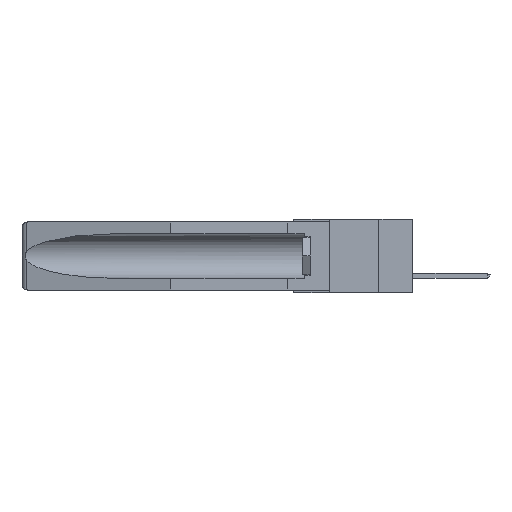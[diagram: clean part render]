
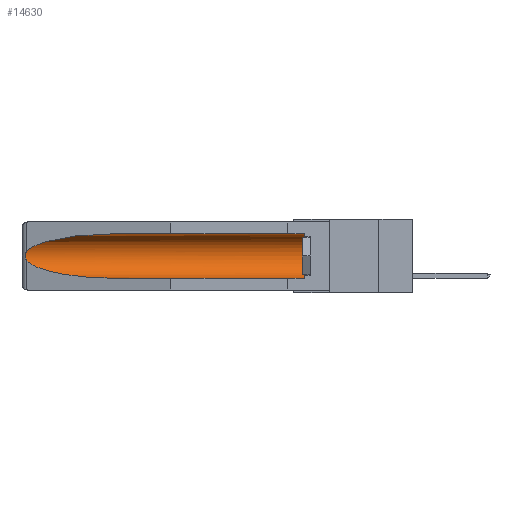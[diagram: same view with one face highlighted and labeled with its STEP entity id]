
A CAD part, left-side view. The second image highlights one B-rep face of the part: STEP entity #14630.
In plain terms, the highlighted cylindrical face has radius 2.857 mm (diameter 5.715 mm), a partial arc.
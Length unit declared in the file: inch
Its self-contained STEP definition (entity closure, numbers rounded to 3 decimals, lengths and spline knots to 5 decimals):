
#13 = CARTESIAN_POINT ( 'NONE',  ( 0.26537, 1.52718, -0.19328 ) ) ;
#518 = DIRECTION ( 'NONE',  ( 0., 0., 1. ) ) ;
#822 = CARTESIAN_POINT ( 'NONE',  ( 0.155, -0.30754, -0.1715 ) ) ;
#1220 = VECTOR ( 'NONE', #3973, 39.37008 ) ;
#1256 = CARTESIAN_POINT ( 'NONE',  ( 0.26537, 1.52718, -0.14972 ) ) ;
#1940 = ORIENTED_EDGE ( 'NONE', *, *, #6004, .T. ) ;
#2351 = ORIENTED_EDGE ( 'NONE', *, *, #6727, .T. ) ;
#2873 = CARTESIAN_POINT ( 'NONE',  ( 0.155, 1.07973, -0.059 ) ) ;
#3004 = CARTESIAN_POINT ( 'NONE',  ( 0.2675, 1.53308, -0.16763 ) ) ;
#3488 = CIRCLE ( 'NONE', #17014, 0.1125 ) ;
#3973 = DIRECTION ( 'NONE',  ( 0., 1., 0. ) ) ;
#4448 = VERTEX_POINT ( 'NONE', #9307 ) ;
#4563 = CARTESIAN_POINT ( 'NONE',  ( 0.26597, 1.52961, -0.15275 ) ) ;
#4626 = CARTESIAN_POINT ( 'NONE',  ( 0.2673, 1.53269, -0.17917 ) ) ;
#4885 = FACE_OUTER_BOUND ( 'NONE', #11073, .T. ) ;
#5135 = LINE ( 'NONE', #11339, #1220 ) ;
#5980 = CARTESIAN_POINT ( 'NONE',  ( 0.26537, 1.52718, -0.19328 ) ) ;
#6004 = EDGE_CURVE ( 'NONE', #4448, #8619, #3488, .T. ) ;
#6390 = CARTESIAN_POINT ( 'NONE',  ( 0.155, 1.07973, -0.284 ) ) ;
#6418 = ORIENTED_EDGE ( 'NONE', *, *, #13402, .T. ) ;
#6426 = CARTESIAN_POINT ( 'NONE',  ( 0.155, 1.07973, -0.284 ) ) ;
#6449 = CARTESIAN_POINT ( 'NONE',  ( 0.21114, 1.30732, -0.284 ) ) ;
#6727 = EDGE_CURVE ( 'NONE', #12605, #17943, #7594, .T. ) ;
#7241 = VERTEX_POINT ( 'NONE', #6426 ) ;
#7555 = CARTESIAN_POINT ( 'NONE',  ( 0.26597, 1.5296, -0.19026 ) ) ;
#7594 = B_SPLINE_CURVE_WITH_KNOTS ( 'NONE', 3,
 ( #7618, #4563, #14870, #11844, #3004, #16428, #4626, #16356, #7555, #5980 ),
 .UNSPECIFIED., .F., .F.,
 ( 4, 2, 2, 2, 4 ),
 ( 0., 0.00029, 0.00058, 0.00087, 0.00117 ),
 .UNSPECIFIED. ) ;
#7618 = CARTESIAN_POINT ( 'NONE',  ( 0.26537, 1.52718, -0.14972 ) ) ;
#8001 = VECTOR ( 'NONE', #18044, 39.37008 ) ;
#8006 = CARTESIAN_POINT ( 'NONE',  ( 0.26537, 1.52718, -0.19328 ) ) ;
#8587 = VERTEX_POINT ( 'NONE', #12379 ) ;
#8619 = VERTEX_POINT ( 'NONE', #9876 ) ;
#8806 = CARTESIAN_POINT ( 'NONE',  ( 0.26537, 1.52718, -0.14972 ) ) ;
#8815 = CYLINDRICAL_SURFACE ( 'NONE', #12055, 0.1125 ) ;
#9232 = CARTESIAN_POINT ( 'NONE',  ( 0.155, 0.126, -0.1715 ) ) ;
#9307 = CARTESIAN_POINT ( 'NONE',  ( 0.155, 0.126, -0.284 ) ) ;
#9475 = EDGE_CURVE ( 'NONE', #4448, #7241, #15582, .T. ) ;
#9541 = EDGE_CURVE ( 'NONE', #17943, #7241, #14062, .T. ) ;
#9876 = CARTESIAN_POINT ( 'NONE',  ( 0.155, 0.126, -0.059 ) ) ;
#10821 = DIRECTION ( 'NONE',  ( 0., -1., 0. ) ) ;
#11073 = EDGE_LOOP ( 'NONE', ( #6418, #2351, #15085, #17212, #1940, #13129 ) ) ;
#11310 = DIRECTION ( 'NONE',  ( 0., 0., 1. ) ) ;
#11339 = CARTESIAN_POINT ( 'NONE',  ( 0.155, -0.30754, -0.059 ) ) ;
#11844 = CARTESIAN_POINT ( 'NONE',  ( 0.2673, 1.5327, -0.16383 ) ) ;
#12055 = AXIS2_PLACEMENT_3D ( 'NONE', #822, #17046, #11310 ) ;
#12379 = CARTESIAN_POINT ( 'NONE',  ( 0.155, 1.07973, -0.059 ) ) ;
#12605 = VERTEX_POINT ( 'NONE', #1256 ) ;
#13129 = ORIENTED_EDGE ( 'NONE', *, *, #14238, .T. ) ;
#13402 = EDGE_CURVE ( 'NONE', #8587, #12605, #16166, .T. ) ;
#14062 =( BOUNDED_CURVE ( )  B_SPLINE_CURVE ( 3, ( #8006, #15325, #6449, #6390 ),
 .UNSPECIFIED., .F., .F. ) 
 B_SPLINE_CURVE_WITH_KNOTS ( ( 4, 4 ),
 ( 0.1948, 1.5708 ),
 .UNSPECIFIED. ) 
 CURVE ( )  GEOMETRIC_REPRESENTATION_ITEM ( )  RATIONAL_B_SPLINE_CURVE ( ( 1., 0.848, 0.848, 1. ) ) 
 REPRESENTATION_ITEM ( '' )  );
#14238 = EDGE_CURVE ( 'NONE', #8619, #8587, #5135, .T. ) ;
#14525 = CARTESIAN_POINT ( 'NONE',  ( 0.21114, 1.30732, -0.059 ) ) ;
#14630 = ADVANCED_FACE ( 'NONE', ( #4885 ), #8815, .F. ) ;
#14870 = CARTESIAN_POINT ( 'NONE',  ( 0.26654, 1.53092, -0.15636 ) ) ;
#15085 = ORIENTED_EDGE ( 'NONE', *, *, #9541, .T. ) ;
#15325 = CARTESIAN_POINT ( 'NONE',  ( 0.25451, 1.48313, -0.24835 ) ) ;
#15582 = LINE ( 'NONE', #17976, #8001 ) ;
#16166 =( BOUNDED_CURVE ( )  B_SPLINE_CURVE ( 3, ( #2873, #14525, #17636, #8806 ),
 .UNSPECIFIED., .F., .F. ) 
 B_SPLINE_CURVE_WITH_KNOTS ( ( 4, 4 ),
 ( 4.71239, 6.08839 ),
 .UNSPECIFIED. ) 
 CURVE ( )  GEOMETRIC_REPRESENTATION_ITEM ( )  RATIONAL_B_SPLINE_CURVE ( ( 1., 0.848, 0.848, 1. ) ) 
 REPRESENTATION_ITEM ( '' )  );
#16356 = CARTESIAN_POINT ( 'NONE',  ( 0.26655, 1.53094, -0.18657 ) ) ;
#16428 = CARTESIAN_POINT ( 'NONE',  ( 0.2675, 1.53308, -0.17534 ) ) ;
#17014 = AXIS2_PLACEMENT_3D ( 'NONE', #9232, #10821, #518 ) ;
#17046 = DIRECTION ( 'NONE',  ( 0., 1., 0. ) ) ;
#17212 = ORIENTED_EDGE ( 'NONE', *, *, #9475, .F. ) ;
#17636 = CARTESIAN_POINT ( 'NONE',  ( 0.25451, 1.48313, -0.09465 ) ) ;
#17943 = VERTEX_POINT ( 'NONE', #13 ) ;
#17976 = CARTESIAN_POINT ( 'NONE',  ( 0.155, -0.30754, -0.284 ) ) ;
#18044 = DIRECTION ( 'NONE',  ( 0., 1., 0. ) ) ;
